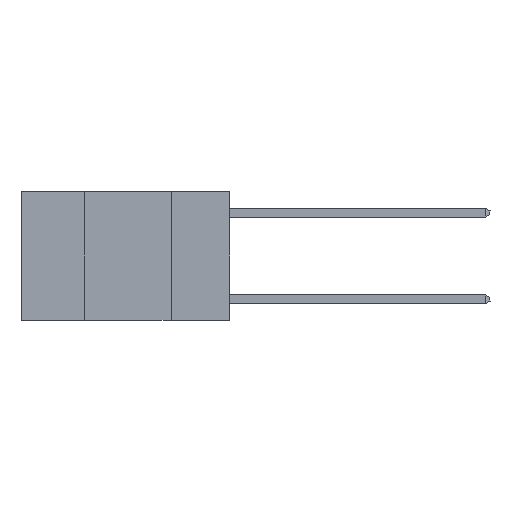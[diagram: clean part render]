
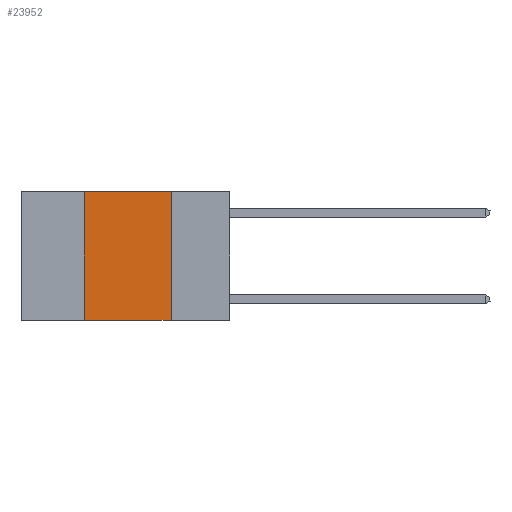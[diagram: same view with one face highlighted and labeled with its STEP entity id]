
A CAD part, left-side view. The second image highlights one B-rep face of the part: STEP entity #23952.
In plain terms, the highlighted planar face has unit normal (-1, 0, 0).
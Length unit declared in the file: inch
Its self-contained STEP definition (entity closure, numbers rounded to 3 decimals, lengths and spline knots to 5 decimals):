
#1094 = ORIENTED_EDGE ( 'NONE', *, *, #7071, .F. ) ;
#1608 = LINE ( 'NONE', #10604, #5662 ) ;
#1724 = VECTOR ( 'NONE', #16392, 39.37008 ) ;
#3048 = DIRECTION ( 'NONE',  ( 0., 0., -1. ) ) ;
#3614 = ORIENTED_EDGE ( 'NONE', *, *, #14063, .F. ) ;
#5180 = CARTESIAN_POINT ( 'NONE',  ( 0., 0.42, 0. ) ) ;
#5662 = VECTOR ( 'NONE', #26420, 39.37008 ) ;
#6449 = CARTESIAN_POINT ( 'NONE',  ( 0., 0.17, 0. ) ) ;
#7071 = EDGE_CURVE ( 'NONE', #21505, #11584, #19214, .T. ) ;
#7186 = CARTESIAN_POINT ( 'NONE',  ( 0., 0.6, 0. ) ) ;
#7470 = PLANE ( 'NONE',  #12950 ) ;
#7694 = LINE ( 'NONE', #11818, #1724 ) ;
#7819 = LINE ( 'NONE', #5180, #23081 ) ;
#8014 = CARTESIAN_POINT ( 'NONE',  ( 0., 0.17, 0. ) ) ;
#10508 = DIRECTION ( 'NONE',  ( 0., 0., -1. ) ) ;
#10604 = CARTESIAN_POINT ( 'NONE',  ( 0., 0.6, 0. ) ) ;
#10802 = EDGE_CURVE ( 'NONE', #24734, #11584, #7694, .T. ) ;
#11584 = VERTEX_POINT ( 'NONE', #15131 ) ;
#11818 = CARTESIAN_POINT ( 'NONE',  ( 0., 0.6, -0.37 ) ) ;
#12950 = AXIS2_PLACEMENT_3D ( 'NONE', #7186, #14538, #3048 ) ;
#14063 = EDGE_CURVE ( 'NONE', #24734, #23953, #7819, .T. ) ;
#14293 = EDGE_CURVE ( 'NONE', #23953, #21505, #1608, .T. ) ;
#14538 = DIRECTION ( 'NONE',  ( 1., 0., 0. ) ) ;
#15131 = CARTESIAN_POINT ( 'NONE',  ( 0., 0.17, -0.37 ) ) ;
#16392 = DIRECTION ( 'NONE',  ( 0., -1., 0. ) ) ;
#18855 = VECTOR ( 'NONE', #10508, 39.37008 ) ;
#19214 = LINE ( 'NONE', #8014, #18855 ) ;
#20496 = CARTESIAN_POINT ( 'NONE',  ( 0., 0.42, -0.37 ) ) ;
#20759 = CARTESIAN_POINT ( 'NONE',  ( 0., 0.42, 0. ) ) ;
#21505 = VERTEX_POINT ( 'NONE', #6449 ) ;
#23081 = VECTOR ( 'NONE', #23763, 39.37008 ) ;
#23140 = FACE_OUTER_BOUND ( 'NONE', #25540, .T. ) ;
#23763 = DIRECTION ( 'NONE',  ( 0., 0., 1. ) ) ;
#23952 = ADVANCED_FACE ( 'NONE', ( #23140 ), #7470, .F. ) ;
#23953 = VERTEX_POINT ( 'NONE', #20759 ) ;
#24734 = VERTEX_POINT ( 'NONE', #20496 ) ;
#25540 = EDGE_LOOP ( 'NONE', ( #1094, #25954, #3614, #27430 ) ) ;
#25954 = ORIENTED_EDGE ( 'NONE', *, *, #14293, .F. ) ;
#26420 = DIRECTION ( 'NONE',  ( 0., -1., 0. ) ) ;
#27430 = ORIENTED_EDGE ( 'NONE', *, *, #10802, .T. ) ;
